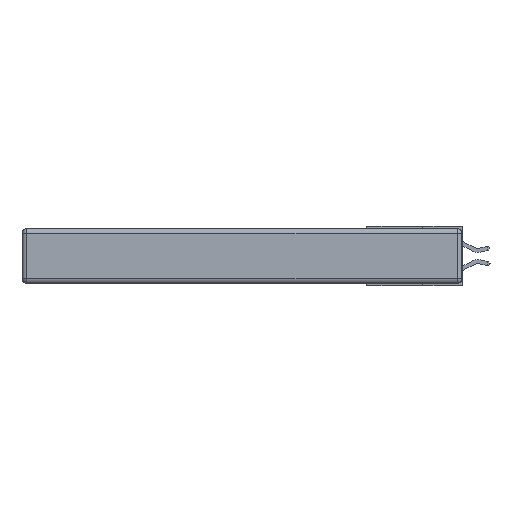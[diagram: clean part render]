
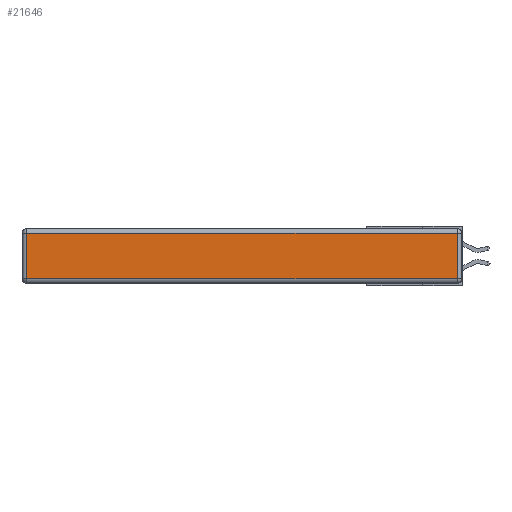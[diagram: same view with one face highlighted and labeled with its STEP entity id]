
A CAD part, left-side view. The second image highlights one B-rep face of the part: STEP entity #21646.
In plain terms, the highlighted planar face has unit normal (-1, 0, 0).
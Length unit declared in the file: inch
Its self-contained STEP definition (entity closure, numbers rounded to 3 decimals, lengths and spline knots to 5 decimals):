
#6 = LINE ( 'NONE', #18955, #20978 ) ;
#28 = EDGE_CURVE ( 'NONE', #10780, #3484, #6, .T. ) ;
#333 = DIRECTION ( 'NONE',  ( -1., 0., 0. ) ) ;
#2196 = PLANE ( 'NONE',  #12149 ) ;
#2246 = VECTOR ( 'NONE', #7695, 39.37008 ) ;
#3253 = FACE_OUTER_BOUND ( 'NONE', #10235, .T. ) ;
#3347 = VECTOR ( 'NONE', #16603, 39.37008 ) ;
#3398 = VERTEX_POINT ( 'NONE', #4487 ) ;
#3484 = VERTEX_POINT ( 'NONE', #20029 ) ;
#4487 = CARTESIAN_POINT ( 'NONE',  ( 0., 2.72, -0.313 ) ) ;
#5394 = VERTEX_POINT ( 'NONE', #20189 ) ;
#7695 = DIRECTION ( 'NONE',  ( 0., 0., -1. ) ) ;
#9027 = EDGE_CURVE ( 'NONE', #3398, #5394, #17440, .T. ) ;
#9641 = ORIENTED_EDGE ( 'NONE', *, *, #21157, .T. ) ;
#9720 = VECTOR ( 'NONE', #14132, 39.37008 ) ;
#10161 = ORIENTED_EDGE ( 'NONE', *, *, #28, .T. ) ;
#10235 = EDGE_LOOP ( 'NONE', ( #11762, #18736, #10161, #9641 ) ) ;
#10641 = CARTESIAN_POINT ( 'NONE',  ( 0., 0.03, -0.343 ) ) ;
#10780 = VERTEX_POINT ( 'NONE', #15425 ) ;
#11066 = CARTESIAN_POINT ( 'NONE',  ( 0., 2.72, -0.343 ) ) ;
#11762 = ORIENTED_EDGE ( 'NONE', *, *, #9027, .T. ) ;
#12149 = AXIS2_PLACEMENT_3D ( 'NONE', #14098, #333, #15874 ) ;
#12888 = LINE ( 'NONE', #11066, #2246 ) ;
#14098 = CARTESIAN_POINT ( 'NONE',  ( 0., 0., -0.343 ) ) ;
#14132 = DIRECTION ( 'NONE',  ( 0., 0., 1. ) ) ;
#15425 = CARTESIAN_POINT ( 'NONE',  ( 0., 0.03, -0.03 ) ) ;
#15874 = DIRECTION ( 'NONE',  ( 0., 0., 1. ) ) ;
#16603 = DIRECTION ( 'NONE',  ( 0., -1., 0. ) ) ;
#16761 = CARTESIAN_POINT ( 'NONE',  ( 0., 0., -0.313 ) ) ;
#17251 = DIRECTION ( 'NONE',  ( 0., 1., 0. ) ) ;
#17440 = LINE ( 'NONE', #16761, #3347 ) ;
#18736 = ORIENTED_EDGE ( 'NONE', *, *, #18759, .T. ) ;
#18752 = LINE ( 'NONE', #10641, #9720 ) ;
#18759 = EDGE_CURVE ( 'NONE', #5394, #10780, #18752, .T. ) ;
#18955 = CARTESIAN_POINT ( 'NONE',  ( 0., 2.75, -0.03 ) ) ;
#20029 = CARTESIAN_POINT ( 'NONE',  ( 0., 2.72, -0.03 ) ) ;
#20189 = CARTESIAN_POINT ( 'NONE',  ( 0., 0.03, -0.313 ) ) ;
#20978 = VECTOR ( 'NONE', #17251, 39.37008 ) ;
#21157 = EDGE_CURVE ( 'NONE', #3484, #3398, #12888, .T. ) ;
#21646 = ADVANCED_FACE ( 'NONE', ( #3253 ), #2196, .T. ) ;
